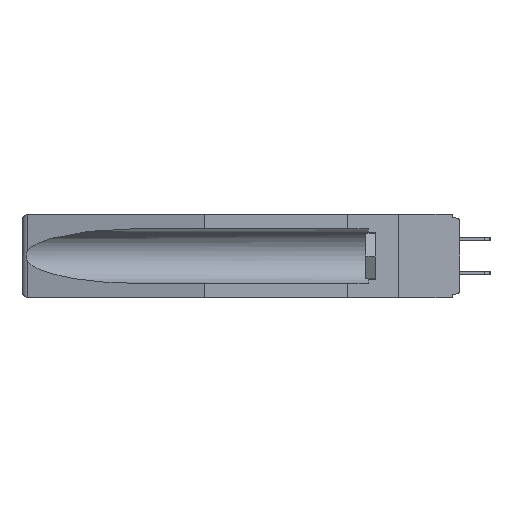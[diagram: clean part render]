
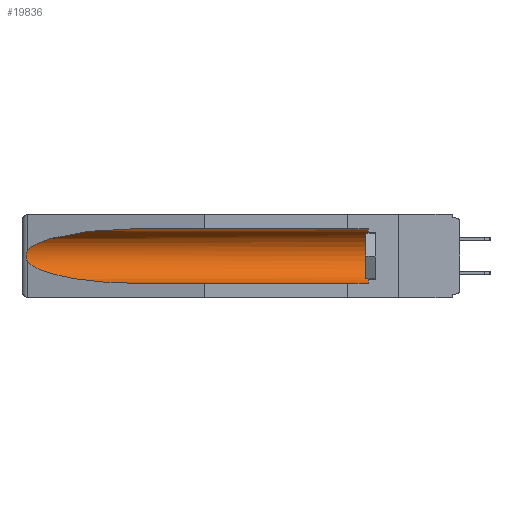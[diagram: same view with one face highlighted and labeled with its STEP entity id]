
A CAD part, left-side view. The second image highlights one B-rep face of the part: STEP entity #19836.
In plain terms, the highlighted cylindrical face has radius 2.857 mm (diameter 5.715 mm), a partial arc.
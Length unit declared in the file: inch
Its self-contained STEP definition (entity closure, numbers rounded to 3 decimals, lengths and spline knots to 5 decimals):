
#1077 = CARTESIAN_POINT ( 'NONE',  ( 0.2675, 1.53308, -0.17534 ) ) ;
#1740 = VECTOR ( 'NONE', #5714, 39.37008 ) ;
#2168 = B_SPLINE_CURVE_WITH_KNOTS ( 'NONE', 3,
 ( #20419, #8291, #25342, #10732, #15597, #1077, #10412, #22465, #7853, #24907 ),
 .UNSPECIFIED., .F., .F.,
 ( 4, 2, 2, 2, 4 ),
 ( 0., 0.00029, 0.00058, 0.00087, 0.00117 ),
 .UNSPECIFIED. ) ;
#2246 = DIRECTION ( 'NONE',  ( 0., -1., 0. ) ) ;
#2318 = EDGE_CURVE ( 'NONE', #10751, #12802, #5431, .T. ) ;
#3289 = CARTESIAN_POINT ( 'NONE',  ( 0.155, -0.30754, -0.059 ) ) ;
#3544 = CARTESIAN_POINT ( 'NONE',  ( 0.155, 0.126, -0.284 ) ) ;
#4889 = DIRECTION ( 'NONE',  ( 0., 0., 1. ) ) ;
#4913 = CYLINDRICAL_SURFACE ( 'NONE', #28009, 0.1125 ) ;
#5431 =( BOUNDED_CURVE ( )  B_SPLINE_CURVE ( 3, ( #14750, #9792, #26741, #19270 ),
 .UNSPECIFIED., .F., .F. ) 
 B_SPLINE_CURVE_WITH_KNOTS ( ( 4, 4 ),
 ( 0.1948, 1.5708 ),
 .UNSPECIFIED. ) 
 CURVE ( )  GEOMETRIC_REPRESENTATION_ITEM ( )  RATIONAL_B_SPLINE_CURVE ( ( 1., 0.848, 0.848, 1. ) ) 
 REPRESENTATION_ITEM ( '' )  );
#5714 = DIRECTION ( 'NONE',  ( 0., 1., 0. ) ) ;
#7853 = CARTESIAN_POINT ( 'NONE',  ( 0.26597, 1.5296, -0.19026 ) ) ;
#8038 = CARTESIAN_POINT ( 'NONE',  ( 0.155, -0.30754, -0.284 ) ) ;
#8291 = CARTESIAN_POINT ( 'NONE',  ( 0.26597, 1.52961, -0.15275 ) ) ;
#8747 = EDGE_CURVE ( 'NONE', #15452, #13943, #21147, .T. ) ;
#8862 = VERTEX_POINT ( 'NONE', #9983 ) ;
#9792 = CARTESIAN_POINT ( 'NONE',  ( 0.25451, 1.48313, -0.24835 ) ) ;
#9983 = CARTESIAN_POINT ( 'NONE',  ( 0.26537, 1.52718, -0.14972 ) ) ;
#10386 = DIRECTION ( 'NONE',  ( 0., 1., 0. ) ) ;
#10412 = CARTESIAN_POINT ( 'NONE',  ( 0.2673, 1.53269, -0.17917 ) ) ;
#10491 = CARTESIAN_POINT ( 'NONE',  ( 0.26537, 1.52718, -0.14972 ) ) ;
#10607 = ORIENTED_EDGE ( 'NONE', *, *, #29592, .T. ) ;
#10732 = CARTESIAN_POINT ( 'NONE',  ( 0.2673, 1.5327, -0.16383 ) ) ;
#10751 = VERTEX_POINT ( 'NONE', #17943 ) ;
#11615 = LINE ( 'NONE', #3289, #1740 ) ;
#11915 = VERTEX_POINT ( 'NONE', #25012 ) ;
#12802 = VERTEX_POINT ( 'NONE', #28549 ) ;
#13808 = EDGE_CURVE ( 'NONE', #8862, #10751, #2168, .T. ) ;
#13943 = VERTEX_POINT ( 'NONE', #16615 ) ;
#14469 = CARTESIAN_POINT ( 'NONE',  ( 0.155, -0.30754, -0.1715 ) ) ;
#14750 = CARTESIAN_POINT ( 'NONE',  ( 0.26537, 1.52718, -0.19328 ) ) ;
#15349 = CARTESIAN_POINT ( 'NONE',  ( 0.155, 1.07973, -0.059 ) ) ;
#15452 = VERTEX_POINT ( 'NONE', #3544 ) ;
#15597 = CARTESIAN_POINT ( 'NONE',  ( 0.2675, 1.53308, -0.16763 ) ) ;
#16615 = CARTESIAN_POINT ( 'NONE',  ( 0.155, 0.126, -0.059 ) ) ;
#16848 = VECTOR ( 'NONE', #10386, 39.37008 ) ;
#17019 = DIRECTION ( 'NONE',  ( 0., 1., 0. ) ) ;
#17417 = ORIENTED_EDGE ( 'NONE', *, *, #24275, .T. ) ;
#17531 = ORIENTED_EDGE ( 'NONE', *, *, #23040, .F. ) ;
#17943 = CARTESIAN_POINT ( 'NONE',  ( 0.26537, 1.52718, -0.19328 ) ) ;
#18030 = CARTESIAN_POINT ( 'NONE',  ( 0.21114, 1.30732, -0.059 ) ) ;
#19270 = CARTESIAN_POINT ( 'NONE',  ( 0.155, 1.07973, -0.284 ) ) ;
#19836 = ADVANCED_FACE ( 'NONE', ( #22863 ), #4913, .F. ) ;
#19950 = ORIENTED_EDGE ( 'NONE', *, *, #8747, .T. ) ;
#20419 = CARTESIAN_POINT ( 'NONE',  ( 0.26537, 1.52718, -0.14972 ) ) ;
#20490 =( BOUNDED_CURVE ( )  B_SPLINE_CURVE ( 3, ( #15349, #18030, #23097, #10491 ),
 .UNSPECIFIED., .F., .F. ) 
 B_SPLINE_CURVE_WITH_KNOTS ( ( 4, 4 ),
 ( 4.71239, 6.08839 ),
 .UNSPECIFIED. ) 
 CURVE ( )  GEOMETRIC_REPRESENTATION_ITEM ( )  RATIONAL_B_SPLINE_CURVE ( ( 1., 0.848, 0.848, 1. ) ) 
 REPRESENTATION_ITEM ( '' )  );
#21147 = CIRCLE ( 'NONE', #25353, 0.1125 ) ;
#21666 = ORIENTED_EDGE ( 'NONE', *, *, #13808, .T. ) ;
#22465 = CARTESIAN_POINT ( 'NONE',  ( 0.26655, 1.53094, -0.18657 ) ) ;
#22571 = EDGE_LOOP ( 'NONE', ( #17417, #21666, #25282, #17531, #19950, #10607 ) ) ;
#22863 = FACE_OUTER_BOUND ( 'NONE', #22571, .T. ) ;
#23040 = EDGE_CURVE ( 'NONE', #15452, #12802, #31313, .T. ) ;
#23097 = CARTESIAN_POINT ( 'NONE',  ( 0.25451, 1.48313, -0.09465 ) ) ;
#24275 = EDGE_CURVE ( 'NONE', #11915, #8862, #20490, .T. ) ;
#24907 = CARTESIAN_POINT ( 'NONE',  ( 0.26537, 1.52718, -0.19328 ) ) ;
#25012 = CARTESIAN_POINT ( 'NONE',  ( 0.155, 1.07973, -0.059 ) ) ;
#25282 = ORIENTED_EDGE ( 'NONE', *, *, #2318, .T. ) ;
#25342 = CARTESIAN_POINT ( 'NONE',  ( 0.26654, 1.53092, -0.15636 ) ) ;
#25353 = AXIS2_PLACEMENT_3D ( 'NONE', #28943, #2246, #29145 ) ;
#26741 = CARTESIAN_POINT ( 'NONE',  ( 0.21114, 1.30732, -0.284 ) ) ;
#28009 = AXIS2_PLACEMENT_3D ( 'NONE', #14469, #17019, #4889 ) ;
#28549 = CARTESIAN_POINT ( 'NONE',  ( 0.155, 1.07973, -0.284 ) ) ;
#28943 = CARTESIAN_POINT ( 'NONE',  ( 0.155, 0.126, -0.1715 ) ) ;
#29145 = DIRECTION ( 'NONE',  ( 0., 0., 1. ) ) ;
#29592 = EDGE_CURVE ( 'NONE', #13943, #11915, #11615, .T. ) ;
#31313 = LINE ( 'NONE', #8038, #16848 ) ;
